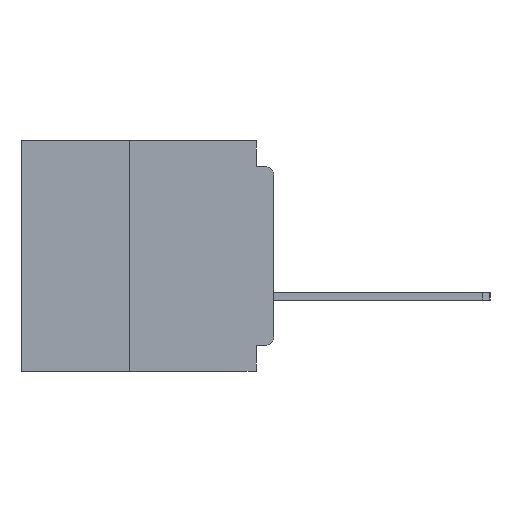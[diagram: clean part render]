
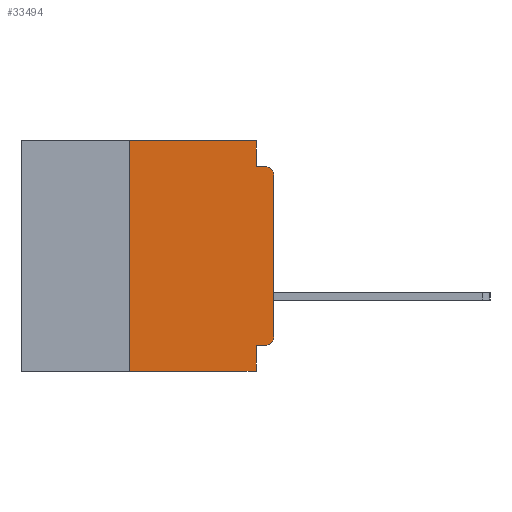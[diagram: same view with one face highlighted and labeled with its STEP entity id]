
A CAD part, left-side view. The second image highlights one B-rep face of the part: STEP entity #33494.
In plain terms, the highlighted planar face has unit normal (-1, 0, 0).
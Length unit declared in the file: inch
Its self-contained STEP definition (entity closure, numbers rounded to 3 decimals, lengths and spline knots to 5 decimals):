
#961 = CARTESIAN_POINT ( 'NONE',  ( 0., 0.031, -0.4 ) ) ;
#1381 = CARTESIAN_POINT ( 'NONE',  ( 0., 0.015, -0.34 ) ) ;
#2539 = DIRECTION ( 'NONE',  ( 0., 0., -1. ) ) ;
#2573 = PLANE ( 'NONE',  #25052 ) ;
#4223 = LINE ( 'NONE', #34981, #27110 ) ;
#5032 = EDGE_CURVE ( 'NONE', #24384, #34167, #15769, .T. ) ;
#5452 = ORIENTED_EDGE ( 'NONE', *, *, #15640, .F. ) ;
#6019 = DIRECTION ( 'NONE',  ( 0., 0., -1. ) ) ;
#6064 = VERTEX_POINT ( 'NONE', #34341 ) ;
#6885 = DIRECTION ( 'NONE',  ( 0., -1., 0. ) ) ;
#7348 = CARTESIAN_POINT ( 'NONE',  ( 0., 0.437, 0. ) ) ;
#8240 = EDGE_CURVE ( 'NONE', #20957, #21934, #26612, .T. ) ;
#8567 = CARTESIAN_POINT ( 'NONE',  ( 0., 0.031, 0. ) ) ;
#8732 = AXIS2_PLACEMENT_3D ( 'NONE', #1381, #33348, #6019 ) ;
#8920 = LINE ( 'NONE', #43344, #30319 ) ;
#9678 = LINE ( 'NONE', #29641, #32512 ) ;
#9941 = EDGE_CURVE ( 'NONE', #6064, #29054, #51794, .T. ) ;
#10119 = EDGE_LOOP ( 'NONE', ( #32226, #44669, #28182, #46121, #22944, #5452, #58383, #13992, #22539, #26162 ) ) ;
#10307 = LINE ( 'NONE', #8567, #33144 ) ;
#11801 = DIRECTION ( 'NONE',  ( 1., 0., 0. ) ) ;
#11950 = DIRECTION ( 'NONE',  ( 0., -1., 0. ) ) ;
#12439 = VECTOR ( 'NONE', #27659, 39.37008 ) ;
#13992 = ORIENTED_EDGE ( 'NONE', *, *, #50092, .F. ) ;
#14128 = DIRECTION ( 'NONE',  ( 0., 0., -1. ) ) ;
#15640 = EDGE_CURVE ( 'NONE', #44395, #20957, #8920, .T. ) ;
#15769 = LINE ( 'NONE', #25481, #39917 ) ;
#18667 = FACE_OUTER_BOUND ( 'NONE', #10119, .T. ) ;
#20034 = VERTEX_POINT ( 'NONE', #961 ) ;
#20485 = EDGE_CURVE ( 'NONE', #21934, #21203, #10307, .T. ) ;
#20717 = DIRECTION ( 'NONE',  ( 0., 1., 0. ) ) ;
#20957 = VERTEX_POINT ( 'NONE', #21126 ) ;
#21126 = CARTESIAN_POINT ( 'NONE',  ( 0., 0.25, 0. ) ) ;
#21203 = VERTEX_POINT ( 'NONE', #54475 ) ;
#21934 = VERTEX_POINT ( 'NONE', #37656 ) ;
#22539 = ORIENTED_EDGE ( 'NONE', *, *, #5032, .F. ) ;
#22944 = ORIENTED_EDGE ( 'NONE', *, *, #8240, .F. ) ;
#23434 = CIRCLE ( 'NONE', #8732, 0.015 ) ;
#24384 = VERTEX_POINT ( 'NONE', #29795 ) ;
#24587 = LINE ( 'NONE', #54850, #12439 ) ;
#25052 = AXIS2_PLACEMENT_3D ( 'NONE', #29758, #11801, #43557 ) ;
#25198 = CARTESIAN_POINT ( 'NONE',  ( 0., 0.25, -0.4 ) ) ;
#25481 = CARTESIAN_POINT ( 'NONE',  ( 0., 0., -0.355 ) ) ;
#25671 = CARTESIAN_POINT ( 'NONE',  ( 0., 0., -0.34 ) ) ;
#26162 = ORIENTED_EDGE ( 'NONE', *, *, #45202, .T. ) ;
#26612 = LINE ( 'NONE', #7348, #47779 ) ;
#27110 = VECTOR ( 'NONE', #39524, 39.37008 ) ;
#27659 = DIRECTION ( 'NONE',  ( 0., -1., 0. ) ) ;
#28182 = ORIENTED_EDGE ( 'NONE', *, *, #56834, .F. ) ;
#29054 = VERTEX_POINT ( 'NONE', #31629 ) ;
#29641 = CARTESIAN_POINT ( 'NONE',  ( 0., 0.437, -0.4 ) ) ;
#29758 = CARTESIAN_POINT ( 'NONE',  ( 0., 0.437, 0. ) ) ;
#29795 = CARTESIAN_POINT ( 'NONE',  ( 0., 0.015, -0.355 ) ) ;
#29930 = DIRECTION ( 'NONE',  ( -1., 0., 0. ) ) ;
#30319 = VECTOR ( 'NONE', #44722, 39.37008 ) ;
#31629 = CARTESIAN_POINT ( 'NONE',  ( 0., 0.015, -0.045 ) ) ;
#32226 = ORIENTED_EDGE ( 'NONE', *, *, #54027, .T. ) ;
#32512 = VECTOR ( 'NONE', #6885, 39.37008 ) ;
#33144 = VECTOR ( 'NONE', #35656, 39.37008 ) ;
#33348 = DIRECTION ( 'NONE',  ( -1., 0., 0. ) ) ;
#33494 = ADVANCED_FACE ( 'NONE', ( #18667 ), #2573, .F. ) ;
#34167 = VERTEX_POINT ( 'NONE', #49587 ) ;
#34341 = CARTESIAN_POINT ( 'NONE',  ( 0., 0., -0.06 ) ) ;
#34981 = CARTESIAN_POINT ( 'NONE',  ( 0., 0., 0. ) ) ;
#35656 = DIRECTION ( 'NONE',  ( 0., 0., -1. ) ) ;
#36939 = VERTEX_POINT ( 'NONE', #25671 ) ;
#37656 = CARTESIAN_POINT ( 'NONE',  ( 0., 0.031, 0. ) ) ;
#39524 = DIRECTION ( 'NONE',  ( 0., 0., 1. ) ) ;
#39917 = VECTOR ( 'NONE', #20717, 39.37008 ) ;
#41327 = CARTESIAN_POINT ( 'NONE',  ( 0., 0.031, -0.4 ) ) ;
#43344 = CARTESIAN_POINT ( 'NONE',  ( 0., 0.25, -0.4 ) ) ;
#43557 = DIRECTION ( 'NONE',  ( 0., 0., -1. ) ) ;
#44056 = AXIS2_PLACEMENT_3D ( 'NONE', #56920, #29930, #2539 ) ;
#44395 = VERTEX_POINT ( 'NONE', #25198 ) ;
#44669 = ORIENTED_EDGE ( 'NONE', *, *, #9941, .T. ) ;
#44722 = DIRECTION ( 'NONE',  ( 0., 0., 1. ) ) ;
#45202 = EDGE_CURVE ( 'NONE', #24384, #36939, #23434, .T. ) ;
#46121 = ORIENTED_EDGE ( 'NONE', *, *, #20485, .F. ) ;
#46525 = EDGE_CURVE ( 'NONE', #44395, #20034, #9678, .T. ) ;
#47464 = VECTOR ( 'NONE', #14128, 39.37008 ) ;
#47779 = VECTOR ( 'NONE', #11950, 39.37008 ) ;
#48884 = LINE ( 'NONE', #41327, #47464 ) ;
#49587 = CARTESIAN_POINT ( 'NONE',  ( 0., 0.031, -0.355 ) ) ;
#50092 = EDGE_CURVE ( 'NONE', #34167, #20034, #48884, .T. ) ;
#51794 = CIRCLE ( 'NONE', #44056, 0.015 ) ;
#54027 = EDGE_CURVE ( 'NONE', #36939, #6064, #4223, .T. ) ;
#54475 = CARTESIAN_POINT ( 'NONE',  ( 0., 0.031, -0.045 ) ) ;
#54850 = CARTESIAN_POINT ( 'NONE',  ( 0., 0., -0.045 ) ) ;
#56834 = EDGE_CURVE ( 'NONE', #21203, #29054, #24587, .T. ) ;
#56920 = CARTESIAN_POINT ( 'NONE',  ( 0., 0.015, -0.06 ) ) ;
#58383 = ORIENTED_EDGE ( 'NONE', *, *, #46525, .T. ) ;
